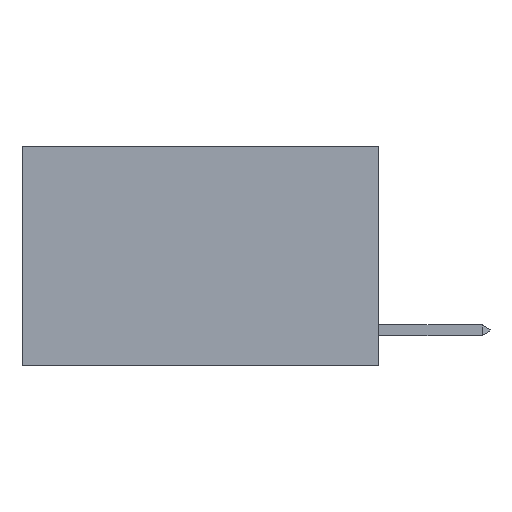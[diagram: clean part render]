
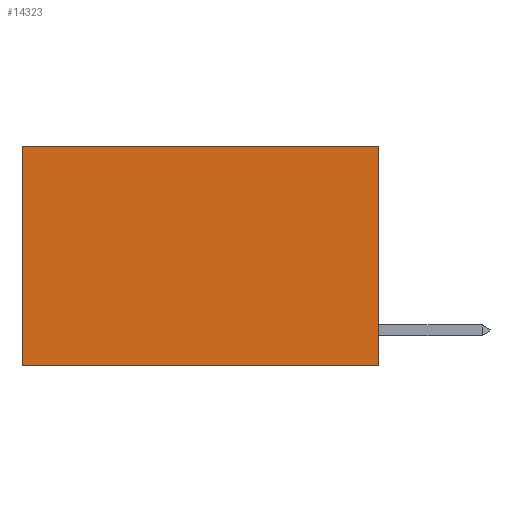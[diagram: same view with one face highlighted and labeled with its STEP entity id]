
A CAD part, left-side view. The second image highlights one B-rep face of the part: STEP entity #14323.
In plain terms, the highlighted planar face has unit normal (-1, 0, 0).
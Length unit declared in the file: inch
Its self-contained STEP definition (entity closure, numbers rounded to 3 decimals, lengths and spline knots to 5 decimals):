
#301 = VECTOR ( 'NONE', #21296, 39.37008 ) ;
#1233 = ORIENTED_EDGE ( 'NONE', *, *, #8482, .F. ) ;
#1263 = DIRECTION ( 'NONE',  ( 0., 0., -1. ) ) ;
#1267 = PLANE ( 'NONE',  #8938 ) ;
#1512 = DIRECTION ( 'NONE',  ( 0., 1., 0. ) ) ;
#3204 = FACE_OUTER_BOUND ( 'NONE', #3618, .T. ) ;
#3330 = VERTEX_POINT ( 'NONE', #15323 ) ;
#3618 = EDGE_LOOP ( 'NONE', ( #4208, #19693, #1233, #5084 ) ) ;
#4208 = ORIENTED_EDGE ( 'NONE', *, *, #16019, .T. ) ;
#4675 = DIRECTION ( 'NONE',  ( 0., 0., -1. ) ) ;
#5084 = ORIENTED_EDGE ( 'NONE', *, *, #18370, .T. ) ;
#6960 = LINE ( 'NONE', #8149, #16157 ) ;
#8149 = CARTESIAN_POINT ( 'NONE',  ( 0.2625, 0., -0.37 ) ) ;
#8482 = EDGE_CURVE ( 'NONE', #21320, #3330, #22488, .T. ) ;
#8938 = AXIS2_PLACEMENT_3D ( 'NONE', #19042, #13765, #15708 ) ;
#10303 = EDGE_CURVE ( 'NONE', #3330, #17174, #6960, .T. ) ;
#13677 = LINE ( 'NONE', #17083, #301 ) ;
#13765 = DIRECTION ( 'NONE',  ( 1., 0., 0. ) ) ;
#13918 = VERTEX_POINT ( 'NONE', #14846 ) ;
#14323 = ADVANCED_FACE ( 'NONE', ( #3204 ), #1267, .F. ) ;
#14339 = CARTESIAN_POINT ( 'NONE',  ( 0.2625, 0., 0. ) ) ;
#14846 = CARTESIAN_POINT ( 'NONE',  ( 0.2625, 0.6, 0. ) ) ;
#15197 = LINE ( 'NONE', #20957, #18526 ) ;
#15323 = CARTESIAN_POINT ( 'NONE',  ( 0.2625, 0., -0.37 ) ) ;
#15674 = CARTESIAN_POINT ( 'NONE',  ( 0.2625, 0.6, -0.37 ) ) ;
#15708 = DIRECTION ( 'NONE',  ( 0., 0., -1. ) ) ;
#16019 = EDGE_CURVE ( 'NONE', #13918, #17174, #15197, .T. ) ;
#16157 = VECTOR ( 'NONE', #1512, 39.37008 ) ;
#17083 = CARTESIAN_POINT ( 'NONE',  ( 0.2625, 0., 0. ) ) ;
#17174 = VERTEX_POINT ( 'NONE', #15674 ) ;
#17808 = VECTOR ( 'NONE', #4675, 39.37008 ) ;
#18370 = EDGE_CURVE ( 'NONE', #21320, #13918, #13677, .T. ) ;
#18526 = VECTOR ( 'NONE', #1263, 39.37008 ) ;
#19042 = CARTESIAN_POINT ( 'NONE',  ( 0.2625, 0., 0. ) ) ;
#19693 = ORIENTED_EDGE ( 'NONE', *, *, #10303, .F. ) ;
#20360 = CARTESIAN_POINT ( 'NONE',  ( 0.2625, 0., 0. ) ) ;
#20957 = CARTESIAN_POINT ( 'NONE',  ( 0.2625, 0.6, 0. ) ) ;
#21296 = DIRECTION ( 'NONE',  ( 0., 1., 0. ) ) ;
#21320 = VERTEX_POINT ( 'NONE', #20360 ) ;
#22488 = LINE ( 'NONE', #14339, #17808 ) ;
